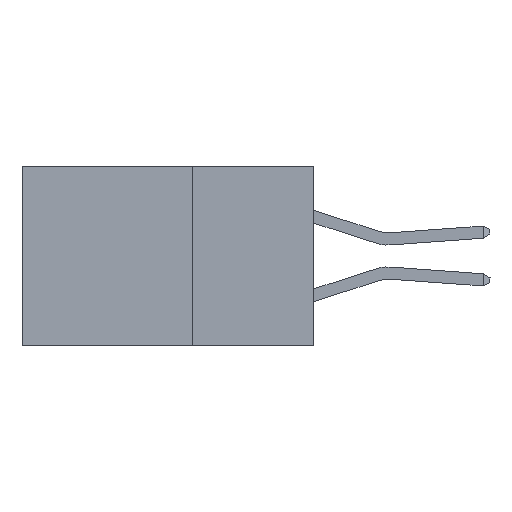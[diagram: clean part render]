
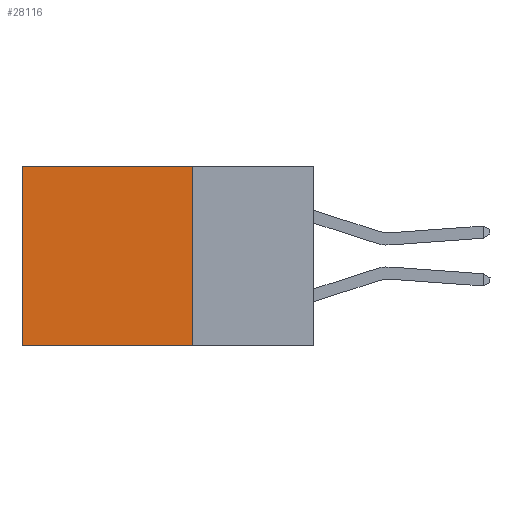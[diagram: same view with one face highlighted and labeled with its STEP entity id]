
A CAD part, left-side view. The second image highlights one B-rep face of the part: STEP entity #28116.
In plain terms, the highlighted planar face has unit normal (-1, 0, 0).
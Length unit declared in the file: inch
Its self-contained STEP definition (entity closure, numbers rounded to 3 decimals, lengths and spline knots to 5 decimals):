
#46 = EDGE_LOOP ( 'NONE', ( #31230, #8775, #4590, #23116 ) ) ;
#1229 = DIRECTION ( 'NONE',  ( 0., 0., -1. ) ) ;
#1469 = CARTESIAN_POINT ( 'NONE',  ( 0.2875, 0.6, -0.37 ) ) ;
#1909 = CARTESIAN_POINT ( 'NONE',  ( 0.2875, 0.25, 0. ) ) ;
#3010 = PLANE ( 'NONE',  #24057 ) ;
#3865 = DIRECTION ( 'NONE',  ( 0., 0., -1. ) ) ;
#4309 = CARTESIAN_POINT ( 'NONE',  ( 0.2875, 0.25, -0.37 ) ) ;
#4590 = ORIENTED_EDGE ( 'NONE', *, *, #12454, .F. ) ;
#4929 = VERTEX_POINT ( 'NONE', #1909 ) ;
#4963 = CARTESIAN_POINT ( 'NONE',  ( 0.2875, 0.6, 0. ) ) ;
#5522 = CARTESIAN_POINT ( 'NONE',  ( 0.2875, 0.25, -0.37 ) ) ;
#7140 = VERTEX_POINT ( 'NONE', #4309 ) ;
#8599 = CARTESIAN_POINT ( 'NONE',  ( 0.2875, 0.25, 0. ) ) ;
#8775 = ORIENTED_EDGE ( 'NONE', *, *, #20642, .F. ) ;
#8800 = VERTEX_POINT ( 'NONE', #1469 ) ;
#8853 = LINE ( 'NONE', #5522, #11086 ) ;
#8986 = VECTOR ( 'NONE', #28356, 39.37008 ) ;
#9097 = VECTOR ( 'NONE', #33371, 39.37008 ) ;
#11086 = VECTOR ( 'NONE', #28767, 39.37008 ) ;
#11578 = CARTESIAN_POINT ( 'NONE',  ( 0.2875, 0.25, 0. ) ) ;
#12259 = VERTEX_POINT ( 'NONE', #14416 ) ;
#12339 = DIRECTION ( 'NONE',  ( 1., 0., 0. ) ) ;
#12454 = EDGE_CURVE ( 'NONE', #4929, #7140, #23080, .T. ) ;
#14416 = CARTESIAN_POINT ( 'NONE',  ( 0.2875, 0.6, 0. ) ) ;
#19448 = FACE_OUTER_BOUND ( 'NONE', #46, .T. ) ;
#20642 = EDGE_CURVE ( 'NONE', #7140, #8800, #8853, .T. ) ;
#21776 = VECTOR ( 'NONE', #1229, 39.37008 ) ;
#23080 = LINE ( 'NONE', #35295, #21776 ) ;
#23116 = ORIENTED_EDGE ( 'NONE', *, *, #25682, .T. ) ;
#24057 = AXIS2_PLACEMENT_3D ( 'NONE', #11578, #12339, #3865 ) ;
#25682 = EDGE_CURVE ( 'NONE', #4929, #12259, #32521, .T. ) ;
#28116 = ADVANCED_FACE ( 'NONE', ( #19448 ), #3010, .F. ) ;
#28356 = DIRECTION ( 'NONE',  ( 0., 1., 0. ) ) ;
#28767 = DIRECTION ( 'NONE',  ( 0., 1., 0. ) ) ;
#29116 = LINE ( 'NONE', #4963, #9097 ) ;
#31230 = ORIENTED_EDGE ( 'NONE', *, *, #36512, .T. ) ;
#32521 = LINE ( 'NONE', #8599, #8986 ) ;
#33371 = DIRECTION ( 'NONE',  ( 0., 0., -1. ) ) ;
#35295 = CARTESIAN_POINT ( 'NONE',  ( 0.2875, 0.25, 0. ) ) ;
#36512 = EDGE_CURVE ( 'NONE', #12259, #8800, #29116, .T. ) ;
